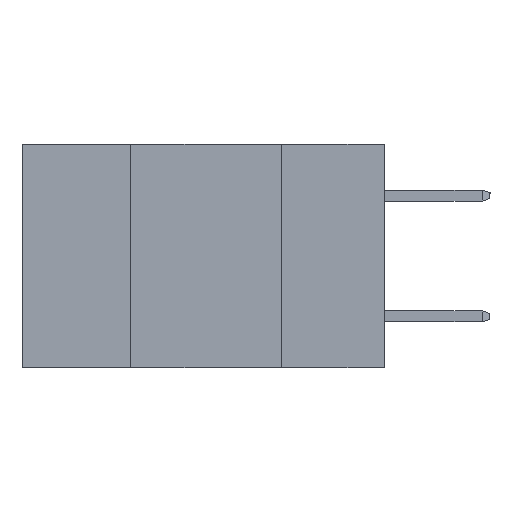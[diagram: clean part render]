
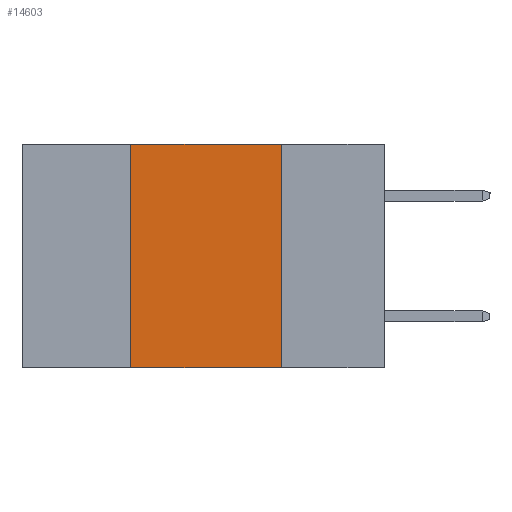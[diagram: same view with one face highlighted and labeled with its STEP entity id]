
A CAD part, left-side view. The second image highlights one B-rep face of the part: STEP entity #14603.
In plain terms, the highlighted planar face has unit normal (-1, 0, 0).
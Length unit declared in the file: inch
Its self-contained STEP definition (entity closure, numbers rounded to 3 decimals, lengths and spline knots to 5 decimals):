
#58 = DIRECTION ( 'NONE',  ( 0., 0., -1. ) ) ;
#392 = CARTESIAN_POINT ( 'NONE',  ( 0., 0.6, 0. ) ) ;
#547 = VECTOR ( 'NONE', #12365, 39.37008 ) ;
#1164 = ORIENTED_EDGE ( 'NONE', *, *, #23088, .T. ) ;
#1325 = EDGE_CURVE ( 'NONE', #7678, #11302, #12389, .T. ) ;
#2151 = VECTOR ( 'NONE', #26798, 39.37008 ) ;
#2230 = ORIENTED_EDGE ( 'NONE', *, *, #15461, .F. ) ;
#3780 = CARTESIAN_POINT ( 'NONE',  ( 0., 0.6, -0.37 ) ) ;
#3923 = LINE ( 'NONE', #3780, #547 ) ;
#4996 = FACE_OUTER_BOUND ( 'NONE', #7022, .T. ) ;
#7022 = EDGE_LOOP ( 'NONE', ( #16914, #2230, #25420, #1164 ) ) ;
#7678 = VERTEX_POINT ( 'NONE', #10837 ) ;
#8201 = CARTESIAN_POINT ( 'NONE',  ( 0., 0.17, -0.37 ) ) ;
#8815 = DIRECTION ( 'NONE',  ( 0., -1., 0. ) ) ;
#10837 = CARTESIAN_POINT ( 'NONE',  ( 0., 0.17, 0. ) ) ;
#11302 = VERTEX_POINT ( 'NONE', #14473 ) ;
#12051 = CARTESIAN_POINT ( 'NONE',  ( 0., 0.42, -0.37 ) ) ;
#12365 = DIRECTION ( 'NONE',  ( 0., -1., 0. ) ) ;
#12389 = LINE ( 'NONE', #8201, #22078 ) ;
#13491 = EDGE_CURVE ( 'NONE', #18654, #19664, #15652, .T. ) ;
#14473 = CARTESIAN_POINT ( 'NONE',  ( 0., 0.17, -0.37 ) ) ;
#14603 = ADVANCED_FACE ( 'NONE', ( #4996 ), #16080, .F. ) ;
#15461 = EDGE_CURVE ( 'NONE', #19664, #7678, #19327, .T. ) ;
#15652 = LINE ( 'NONE', #12051, #2151 ) ;
#15667 = CARTESIAN_POINT ( 'NONE',  ( 0., 0.6, 0. ) ) ;
#16080 = PLANE ( 'NONE',  #25913 ) ;
#16914 = ORIENTED_EDGE ( 'NONE', *, *, #1325, .F. ) ;
#18654 = VERTEX_POINT ( 'NONE', #23025 ) ;
#19327 = LINE ( 'NONE', #392, #20245 ) ;
#19664 = VERTEX_POINT ( 'NONE', #23091 ) ;
#19665 = DIRECTION ( 'NONE',  ( 1., 0., 0. ) ) ;
#20245 = VECTOR ( 'NONE', #8815, 39.37008 ) ;
#22078 = VECTOR ( 'NONE', #58, 39.37008 ) ;
#23025 = CARTESIAN_POINT ( 'NONE',  ( 0., 0.42, -0.37 ) ) ;
#23088 = EDGE_CURVE ( 'NONE', #18654, #11302, #3923, .T. ) ;
#23091 = CARTESIAN_POINT ( 'NONE',  ( 0., 0.42, 0. ) ) ;
#23933 = DIRECTION ( 'NONE',  ( 0., 0., -1. ) ) ;
#25420 = ORIENTED_EDGE ( 'NONE', *, *, #13491, .F. ) ;
#25913 = AXIS2_PLACEMENT_3D ( 'NONE', #15667, #19665, #23933 ) ;
#26798 = DIRECTION ( 'NONE',  ( 0., 0., 1. ) ) ;
